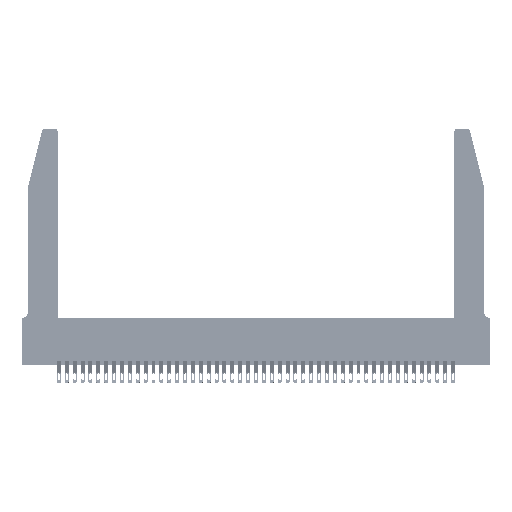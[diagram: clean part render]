
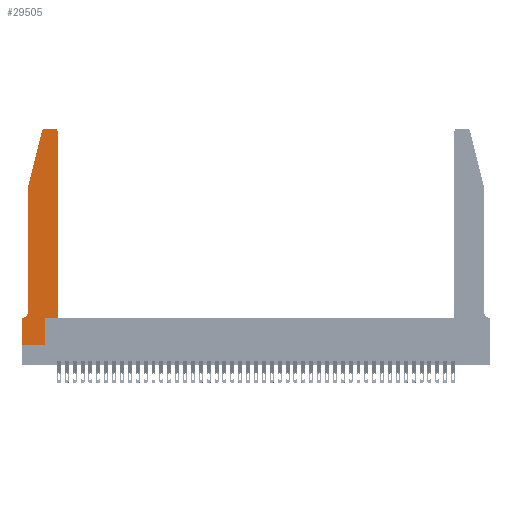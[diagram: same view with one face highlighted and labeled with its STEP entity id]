
A CAD part, top view. The second image highlights one B-rep face of the part: STEP entity #29505.
In plain terms, the highlighted planar face has unit normal (0, 0, 1).
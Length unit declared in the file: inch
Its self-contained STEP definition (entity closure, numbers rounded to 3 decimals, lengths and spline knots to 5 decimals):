
#36 = ORIENTED_EDGE ( 'NONE', *, *, #26835, .T. ) ;
#116 = VERTEX_POINT ( 'NONE', #42948 ) ;
#372 = VERTEX_POINT ( 'NONE', #2486 ) ;
#600 = ORIENTED_EDGE ( 'NONE', *, *, #3740, .T. ) ;
#601 = ORIENTED_EDGE ( 'NONE', *, *, #9283, .T. ) ;
#798 = EDGE_CURVE ( 'NONE', #1501, #372, #4033, .T. ) ;
#846 = PLANE ( 'NONE',  #23795 ) ;
#974 = CARTESIAN_POINT ( 'NONE',  ( 0.0755, 2., 0.37 ) ) ;
#1044 = CARTESIAN_POINT ( 'NONE',  ( 0., 0., 0.37 ) ) ;
#1381 = VERTEX_POINT ( 'NONE', #32160 ) ;
#1501 = VERTEX_POINT ( 'NONE', #25975 ) ;
#2486 = CARTESIAN_POINT ( 'NONE',  ( 0.0055, 0.35, 0.37 ) ) ;
#2487 = VERTEX_POINT ( 'NONE', #34669 ) ;
#3740 = EDGE_CURVE ( 'NONE', #16742, #29139, #42893, .T. ) ;
#3928 = ORIENTED_EDGE ( 'NONE', *, *, #41051, .T. ) ;
#4033 = CIRCLE ( 'NONE', #24869, 0.07 ) ;
#4278 = DIRECTION ( 'NONE',  ( 1., 0., 0. ) ) ;
#4363 = DIRECTION ( 'NONE',  ( 0., 0., 1. ) ) ;
#4453 = LINE ( 'NONE', #974, #12577 ) ;
#4526 = LINE ( 'NONE', #21360, #23767 ) ;
#5114 = CARTESIAN_POINT ( 'NONE',  ( 0.284, 2.72, 0.37 ) ) ;
#5329 = ORIENTED_EDGE ( 'NONE', *, *, #41634, .T. ) ;
#5736 = CARTESIAN_POINT ( 'NONE',  ( 0.4505, 0.35, 0.37 ) ) ;
#5889 = CARTESIAN_POINT ( 'NONE',  ( 0.0755, 2., 0.37 ) ) ;
#7008 = VECTOR ( 'NONE', #13377, 39.37008 ) ;
#7149 = LINE ( 'NONE', #34215, #24180 ) ;
#7846 = ORIENTED_EDGE ( 'NONE', *, *, #8358, .T. ) ;
#8358 = EDGE_CURVE ( 'NONE', #2487, #27267, #21152, .T. ) ;
#8629 = DIRECTION ( 'NONE',  ( 1., 0., 0. ) ) ;
#9283 = EDGE_CURVE ( 'NONE', #28904, #2487, #4526, .T. ) ;
#9556 = AXIS2_PLACEMENT_3D ( 'NONE', #5114, #28887, #8629 ) ;
#10779 = CIRCLE ( 'NONE', #9556, 0.03 ) ;
#11666 = CARTESIAN_POINT ( 'NONE',  ( 0.0055, 0.42, 0.37 ) ) ;
#12337 = VECTOR ( 'NONE', #24176, 39.37008 ) ;
#12438 = ORIENTED_EDGE ( 'NONE', *, *, #23004, .T. ) ;
#12577 = VECTOR ( 'NONE', #14909, 39.37008 ) ;
#12884 = LINE ( 'NONE', #22966, #38613 ) ;
#13111 = CARTESIAN_POINT ( 'NONE',  ( 0., 0., 0.37 ) ) ;
#13321 = CARTESIAN_POINT ( 'NONE',  ( 0.25487, 2.72718, 0.37 ) ) ;
#13377 = DIRECTION ( 'NONE',  ( 0., 1., 0. ) ) ;
#13448 = LINE ( 'NONE', #20820, #12337 ) ;
#14438 = CARTESIAN_POINT ( 'NONE',  ( 0.0755, 2., 0.37 ) ) ;
#14909 = DIRECTION ( 'NONE',  ( 0., -1., 0. ) ) ;
#15148 = DIRECTION ( 'NONE',  ( -1., 0., 0. ) ) ;
#15158 = VECTOR ( 'NONE', #29766, 39.37008 ) ;
#15452 = DIRECTION ( 'NONE',  ( 0., 0., 1. ) ) ;
#16644 = FACE_OUTER_BOUND ( 'NONE', #27301, .T. ) ;
#16742 = VERTEX_POINT ( 'NONE', #5736 ) ;
#16765 = VERTEX_POINT ( 'NONE', #5889 ) ;
#17475 = ORIENTED_EDGE ( 'NONE', *, *, #23192, .T. ) ;
#17877 = DIRECTION ( 'NONE',  ( -0.239, -0.971, 0. ) ) ;
#17929 = VERTEX_POINT ( 'NONE', #32337 ) ;
#18303 = VERTEX_POINT ( 'NONE', #13321 ) ;
#19306 = CIRCLE ( 'NONE', #34530, 0.03 ) ;
#19824 = CARTESIAN_POINT ( 'NONE',  ( 0.2865, 0.35, 0.37 ) ) ;
#19909 = ORIENTED_EDGE ( 'NONE', *, *, #798, .T. ) ;
#20549 = DIRECTION ( 'NONE',  ( -1., 0., 0. ) ) ;
#20820 = CARTESIAN_POINT ( 'NONE',  ( 0.0755, 0.35, 0.37 ) ) ;
#21014 = ORIENTED_EDGE ( 'NONE', *, *, #39509, .T. ) ;
#21152 = LINE ( 'NONE', #19824, #22199 ) ;
#21360 = CARTESIAN_POINT ( 'NONE',  ( 0., 0., 0.37 ) ) ;
#22199 = VECTOR ( 'NONE', #26378, 39.37008 ) ;
#22966 = CARTESIAN_POINT ( 'NONE',  ( 0.4505, 0.35, 0.37 ) ) ;
#23004 = EDGE_CURVE ( 'NONE', #29139, #116, #19306, .T. ) ;
#23104 = DIRECTION ( 'NONE',  ( 1., 0., 0. ) ) ;
#23192 = EDGE_CURVE ( 'NONE', #27267, #16742, #12884, .T. ) ;
#23767 = VECTOR ( 'NONE', #4278, 39.37008 ) ;
#23795 = AXIS2_PLACEMENT_3D ( 'NONE', #24790, #4363, #28154 ) ;
#24176 = DIRECTION ( 'NONE',  ( -1., 0., 0. ) ) ;
#24180 = VECTOR ( 'NONE', #20549, 39.37008 ) ;
#24790 = CARTESIAN_POINT ( 'NONE',  ( 0., 0.35, 0.37 ) ) ;
#24869 = AXIS2_PLACEMENT_3D ( 'NONE', #11666, #35230, #15148 ) ;
#25142 = LINE ( 'NONE', #13111, #15158 ) ;
#25975 = CARTESIAN_POINT ( 'NONE',  ( 0.0755, 0.42, 0.37 ) ) ;
#26130 = CARTESIAN_POINT ( 'NONE',  ( 0.4505, 2.72, 0.37 ) ) ;
#26378 = DIRECTION ( 'NONE',  ( 0., 1., 0. ) ) ;
#26835 = EDGE_CURVE ( 'NONE', #16765, #1501, #4453, .T. ) ;
#27057 = LINE ( 'NONE', #14438, #43814 ) ;
#27267 = VERTEX_POINT ( 'NONE', #33045 ) ;
#27301 = EDGE_LOOP ( 'NONE', ( #21014, #3928, #35030, #36, #19909, #5329, #30759, #601, #7846, #17475, #600, #12438 ) ) ;
#28154 = DIRECTION ( 'NONE',  ( 1., 0., 0. ) ) ;
#28887 = DIRECTION ( 'NONE',  ( 0., 0., 1. ) ) ;
#28904 = VERTEX_POINT ( 'NONE', #1044 ) ;
#29139 = VERTEX_POINT ( 'NONE', #26130 ) ;
#29505 = ADVANCED_FACE ( 'NONE', ( #16644 ), #846, .T. ) ;
#29766 = DIRECTION ( 'NONE',  ( 0., -1., 0. ) ) ;
#30759 = ORIENTED_EDGE ( 'NONE', *, *, #32312, .T. ) ;
#30782 = EDGE_CURVE ( 'NONE', #18303, #16765, #27057, .T. ) ;
#32160 = CARTESIAN_POINT ( 'NONE',  ( 0., 0.35, 0.37 ) ) ;
#32312 = EDGE_CURVE ( 'NONE', #1381, #28904, #25142, .T. ) ;
#32337 = CARTESIAN_POINT ( 'NONE',  ( 0.284, 2.75, 0.37 ) ) ;
#33045 = CARTESIAN_POINT ( 'NONE',  ( 0.2865, 0.35, 0.37 ) ) ;
#34215 = CARTESIAN_POINT ( 'NONE',  ( 0.2605, 2.75, 0.37 ) ) ;
#34530 = AXIS2_PLACEMENT_3D ( 'NONE', #35532, #15452, #38883 ) ;
#34669 = CARTESIAN_POINT ( 'NONE',  ( 0.2865, 0., 0.37 ) ) ;
#35030 = ORIENTED_EDGE ( 'NONE', *, *, #30782, .T. ) ;
#35230 = DIRECTION ( 'NONE',  ( 0., 0., -1. ) ) ;
#35532 = CARTESIAN_POINT ( 'NONE',  ( 0.4205, 2.72, 0.37 ) ) ;
#36838 = CARTESIAN_POINT ( 'NONE',  ( 0.4505, 0.35, 0.37 ) ) ;
#38613 = VECTOR ( 'NONE', #23104, 39.37008 ) ;
#38883 = DIRECTION ( 'NONE',  ( 1., 0., 0. ) ) ;
#39509 = EDGE_CURVE ( 'NONE', #116, #17929, #7149, .T. ) ;
#41051 = EDGE_CURVE ( 'NONE', #17929, #18303, #10779, .T. ) ;
#41634 = EDGE_CURVE ( 'NONE', #372, #1381, #13448, .T. ) ;
#42893 = LINE ( 'NONE', #36838, #7008 ) ;
#42948 = CARTESIAN_POINT ( 'NONE',  ( 0.4205, 2.75, 0.37 ) ) ;
#43814 = VECTOR ( 'NONE', #17877, 39.37008 ) ;
